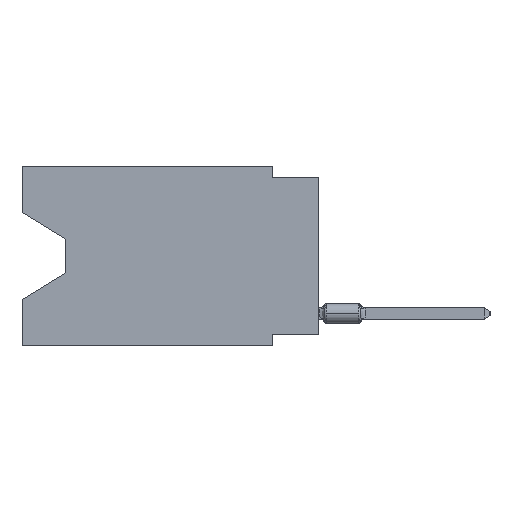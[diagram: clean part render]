
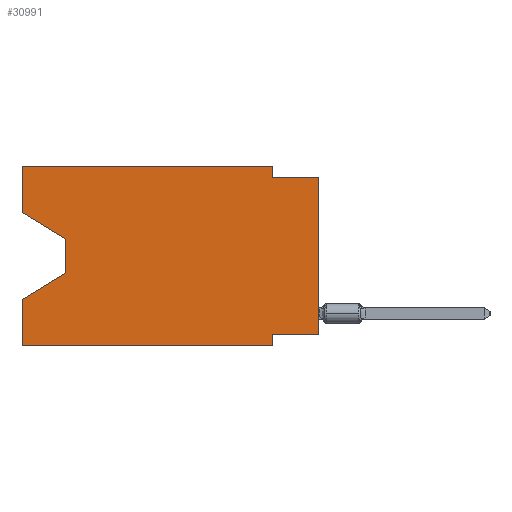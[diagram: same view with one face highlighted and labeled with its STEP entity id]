
A CAD part, left-side view. The second image highlights one B-rep face of the part: STEP entity #30991.
In plain terms, the highlighted planar face has unit normal (-1, 0, 0).
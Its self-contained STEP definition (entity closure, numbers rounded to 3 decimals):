
#124 = VECTOR ( 'NONE', #33523, 1000. ) ;
#484 = LINE ( 'NONE', #48820, #3081 ) ;
#2787 = CARTESIAN_POINT ( 'NONE',  ( 0., 16.383, 0. ) ) ;
#3081 = VECTOR ( 'NONE', #43801, 1000. ) ;
#3746 = EDGE_CURVE ( 'NONE', #38755, #12956, #4338, .T. ) ;
#4338 = LINE ( 'NONE', #6483, #5438 ) ;
#4980 = CARTESIAN_POINT ( 'NONE',  ( 0., 2.54, 0. ) ) ;
#5283 = VERTEX_POINT ( 'NONE', #54835 ) ;
#5438 = VECTOR ( 'NONE', #29443, 1000. ) ;
#5947 = VECTOR ( 'NONE', #17790, 1000. ) ;
#6170 = DIRECTION ( 'NONE',  ( 0., -1., 0. ) ) ;
#6483 = CARTESIAN_POINT ( 'NONE',  ( 0., 0., 0. ) ) ;
#9050 = ORIENTED_EDGE ( 'NONE', *, *, #31759, .F. ) ;
#9131 = EDGE_LOOP ( 'NONE', ( #13711, #32607, #49509, #35844, #54468, #57040, #60205, #27354, #55522, #25275, #16715, #9050 ) ) ;
#10269 = CARTESIAN_POINT ( 'NONE',  ( 0., 13.97, -5.893 ) ) ;
#10391 = CARTESIAN_POINT ( 'NONE',  ( 0., 16.383, 0. ) ) ;
#12956 = VERTEX_POINT ( 'NONE', #37900 ) ;
#12974 = VERTEX_POINT ( 'NONE', #43824 ) ;
#13711 = ORIENTED_EDGE ( 'NONE', *, *, #31481, .T. ) ;
#15404 = PLANE ( 'NONE',  #49014 ) ;
#15952 = VECTOR ( 'NONE', #39772, 1000. ) ;
#16715 = ORIENTED_EDGE ( 'NONE', *, *, #52864, .F. ) ;
#17715 = CARTESIAN_POINT ( 'NONE',  ( 0., 13.97, -4.013 ) ) ;
#17790 = DIRECTION ( 'NONE',  ( 0., 0., -1. ) ) ;
#18547 = VERTEX_POINT ( 'NONE', #4980 ) ;
#19565 = CARTESIAN_POINT ( 'NONE',  ( 0., 2.54, -9.906 ) ) ;
#20244 = CARTESIAN_POINT ( 'NONE',  ( 0., 0., -0.635 ) ) ;
#20940 = LINE ( 'NONE', #30678, #15952 ) ;
#22639 = CARTESIAN_POINT ( 'NONE',  ( 0., 2.54, 0. ) ) ;
#23449 = CARTESIAN_POINT ( 'NONE',  ( 0., 16.383, -9.906 ) ) ;
#24509 = FACE_OUTER_BOUND ( 'NONE', #9131, .T. ) ;
#24594 = LINE ( 'NONE', #39017, #58080 ) ;
#25202 = VECTOR ( 'NONE', #32302, 1000. ) ;
#25275 = ORIENTED_EDGE ( 'NONE', *, *, #46280, .F. ) ;
#25509 = CARTESIAN_POINT ( 'NONE',  ( 0., 13.97, -4.013 ) ) ;
#26579 = VERTEX_POINT ( 'NONE', #44047 ) ;
#27354 = ORIENTED_EDGE ( 'NONE', *, *, #3746, .T. ) ;
#28797 = VERTEX_POINT ( 'NONE', #23449 ) ;
#29443 = DIRECTION ( 'NONE',  ( 0., 0., 1. ) ) ;
#29741 = LINE ( 'NONE', #10269, #124 ) ;
#29826 = CARTESIAN_POINT ( 'NONE',  ( 0., 16.383, 0. ) ) ;
#30678 = CARTESIAN_POINT ( 'NONE',  ( 0., 16.383, -2.546 ) ) ;
#30807 = DIRECTION ( 'NONE',  ( 0., 0., -1. ) ) ;
#30991 = ADVANCED_FACE ( 'NONE', ( #24509 ), #15404, .F. ) ;
#31481 = EDGE_CURVE ( 'NONE', #5283, #34814, #20940, .T. ) ;
#31609 = EDGE_CURVE ( 'NONE', #12974, #48277, #51686, .T. ) ;
#31759 = EDGE_CURVE ( 'NONE', #5283, #35911, #24594, .T. ) ;
#32302 = DIRECTION ( 'NONE',  ( 0., 0., 1. ) ) ;
#32607 = ORIENTED_EDGE ( 'NONE', *, *, #51335, .T. ) ;
#33523 = DIRECTION ( 'NONE',  ( 0., 0.855, -0.519 ) ) ;
#33861 = EDGE_CURVE ( 'NONE', #26579, #35558, #29741, .T. ) ;
#34031 = CARTESIAN_POINT ( 'NONE',  ( 0., 0., -9.271 ) ) ;
#34459 = LINE ( 'NONE', #34755, #51524 ) ;
#34546 = DIRECTION ( 'NONE',  ( 1., 0., 0. ) ) ;
#34755 = CARTESIAN_POINT ( 'NONE',  ( 0., 16.383, -9.906 ) ) ;
#34814 = VERTEX_POINT ( 'NONE', #25509 ) ;
#35252 = EDGE_CURVE ( 'NONE', #28797, #35558, #36406, .T. ) ;
#35558 = VERTEX_POINT ( 'NONE', #48879 ) ;
#35844 = ORIENTED_EDGE ( 'NONE', *, *, #35252, .F. ) ;
#35911 = VERTEX_POINT ( 'NONE', #61658 ) ;
#36406 = LINE ( 'NONE', #2787, #25202 ) ;
#36678 = VECTOR ( 'NONE', #30807, 1000. ) ;
#37502 = LINE ( 'NONE', #17715, #59141 ) ;
#37900 = CARTESIAN_POINT ( 'NONE',  ( 0., 0., -0.635 ) ) ;
#38755 = VERTEX_POINT ( 'NONE', #34031 ) ;
#38957 = DIRECTION ( 'NONE',  ( 0., -1., 0. ) ) ;
#39017 = CARTESIAN_POINT ( 'NONE',  ( 0., 16.383, 0. ) ) ;
#39772 = DIRECTION ( 'NONE',  ( 0., -0.855, -0.519 ) ) ;
#39868 = LINE ( 'NONE', #10391, #49217 ) ;
#41467 = LINE ( 'NONE', #22639, #36678 ) ;
#43801 = DIRECTION ( 'NONE',  ( 0., 1., 0. ) ) ;
#43824 = CARTESIAN_POINT ( 'NONE',  ( 0., 2.54, -9.271 ) ) ;
#44047 = CARTESIAN_POINT ( 'NONE',  ( 0., 13.97, -5.893 ) ) ;
#44553 = DIRECTION ( 'NONE',  ( 0., 0., -1. ) ) ;
#44981 = EDGE_CURVE ( 'NONE', #28797, #48277, #34459, .T. ) ;
#46069 = VECTOR ( 'NONE', #58545, 1000. ) ;
#46280 = EDGE_CURVE ( 'NONE', #18547, #56809, #41467, .T. ) ;
#47865 = LINE ( 'NONE', #20244, #46069 ) ;
#48277 = VERTEX_POINT ( 'NONE', #52527 ) ;
#48820 = CARTESIAN_POINT ( 'NONE',  ( 0., 0., -9.271 ) ) ;
#48879 = CARTESIAN_POINT ( 'NONE',  ( 0., 16.383, -7.36 ) ) ;
#49014 = AXIS2_PLACEMENT_3D ( 'NONE', #29826, #34546, #44553 ) ;
#49217 = VECTOR ( 'NONE', #38957, 1000. ) ;
#49509 = ORIENTED_EDGE ( 'NONE', *, *, #33861, .T. ) ;
#50984 = DIRECTION ( 'NONE',  ( 0., 0., -1. ) ) ;
#51335 = EDGE_CURVE ( 'NONE', #34814, #26579, #37502, .T. ) ;
#51524 = VECTOR ( 'NONE', #6170, 1000. ) ;
#51686 = LINE ( 'NONE', #19565, #5947 ) ;
#52236 = EDGE_CURVE ( 'NONE', #38755, #12974, #484, .T. ) ;
#52527 = CARTESIAN_POINT ( 'NONE',  ( 0., 2.54, -9.906 ) ) ;
#52864 = EDGE_CURVE ( 'NONE', #35911, #18547, #39868, .T. ) ;
#53619 = CARTESIAN_POINT ( 'NONE',  ( 0., 2.54, -0.635 ) ) ;
#54468 = ORIENTED_EDGE ( 'NONE', *, *, #44981, .T. ) ;
#54835 = CARTESIAN_POINT ( 'NONE',  ( 0., 16.383, -2.546 ) ) ;
#55522 = ORIENTED_EDGE ( 'NONE', *, *, #56641, .F. ) ;
#56641 = EDGE_CURVE ( 'NONE', #56809, #12956, #47865, .T. ) ;
#56809 = VERTEX_POINT ( 'NONE', #53619 ) ;
#57040 = ORIENTED_EDGE ( 'NONE', *, *, #31609, .F. ) ;
#58080 = VECTOR ( 'NONE', #58176, 1000. ) ;
#58176 = DIRECTION ( 'NONE',  ( 0., 0., 1. ) ) ;
#58545 = DIRECTION ( 'NONE',  ( 0., -1., 0. ) ) ;
#59141 = VECTOR ( 'NONE', #50984, 1000. ) ;
#60205 = ORIENTED_EDGE ( 'NONE', *, *, #52236, .F. ) ;
#61658 = CARTESIAN_POINT ( 'NONE',  ( 0., 16.383, 0. ) ) ;
